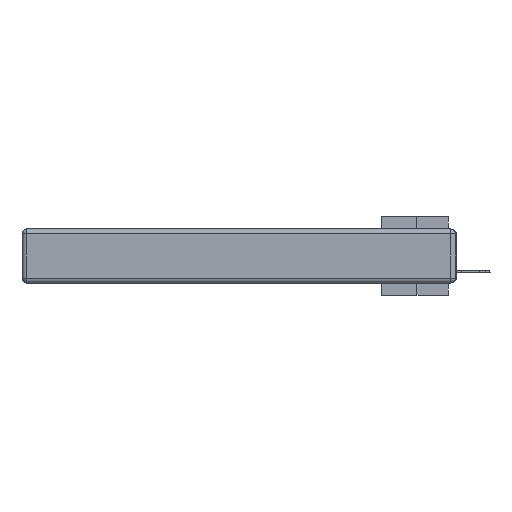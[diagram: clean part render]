
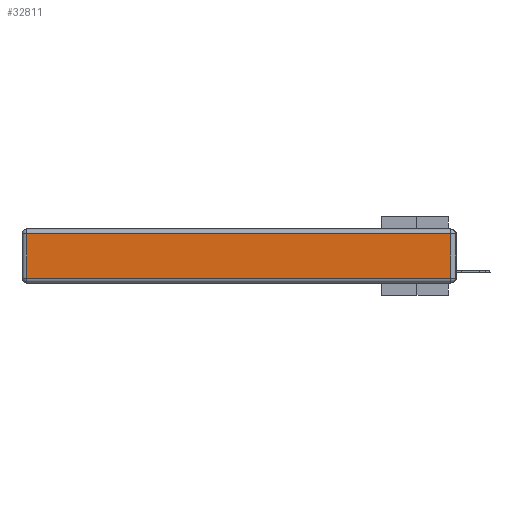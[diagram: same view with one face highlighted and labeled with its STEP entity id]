
A CAD part, left-side view. The second image highlights one B-rep face of the part: STEP entity #32811.
In plain terms, the highlighted planar face has unit normal (-1, 0, 0).
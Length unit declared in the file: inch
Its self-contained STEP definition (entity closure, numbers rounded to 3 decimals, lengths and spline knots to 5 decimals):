
#587 = ORIENTED_EDGE ( 'NONE', *, *, #30968, .T. ) ;
#1299 = EDGE_LOOP ( 'NONE', ( #3835, #18784, #19781, #587 ) ) ;
#2962 = CARTESIAN_POINT ( 'NONE',  ( 0., 0.03, -0.03 ) ) ;
#3835 = ORIENTED_EDGE ( 'NONE', *, *, #29641, .T. ) ;
#3884 = VERTEX_POINT ( 'NONE', #15268 ) ;
#4155 = LINE ( 'NONE', #10941, #34475 ) ;
#4828 = EDGE_CURVE ( 'NONE', #31026, #12802, #4155, .T. ) ;
#4830 = VECTOR ( 'NONE', #8512, 39.37008 ) ;
#5621 = EDGE_CURVE ( 'NONE', #3884, #31026, #7316, .T. ) ;
#7316 = LINE ( 'NONE', #24597, #7793 ) ;
#7793 = VECTOR ( 'NONE', #30874, 39.37008 ) ;
#8512 = DIRECTION ( 'NONE',  ( 0., -1., 0. ) ) ;
#8886 = CARTESIAN_POINT ( 'NONE',  ( 0., 0., -0.313 ) ) ;
#9136 = PLANE ( 'NONE',  #17947 ) ;
#10783 = LINE ( 'NONE', #8886, #4830 ) ;
#10941 = CARTESIAN_POINT ( 'NONE',  ( 0., 2.75, -0.03 ) ) ;
#12802 = VERTEX_POINT ( 'NONE', #35572 ) ;
#13892 = VECTOR ( 'NONE', #23883, 39.37008 ) ;
#13922 = VERTEX_POINT ( 'NONE', #28902 ) ;
#14684 = DIRECTION ( 'NONE',  ( 0., 0., 1. ) ) ;
#15268 = CARTESIAN_POINT ( 'NONE',  ( 0., 0.03, -0.313 ) ) ;
#16967 = DIRECTION ( 'NONE',  ( 0., 1., 0. ) ) ;
#17947 = AXIS2_PLACEMENT_3D ( 'NONE', #32385, #26632, #14684 ) ;
#18784 = ORIENTED_EDGE ( 'NONE', *, *, #5621, .T. ) ;
#19781 = ORIENTED_EDGE ( 'NONE', *, *, #4828, .T. ) ;
#23883 = DIRECTION ( 'NONE',  ( 0., 0., -1. ) ) ;
#24597 = CARTESIAN_POINT ( 'NONE',  ( 0., 0.03, -0.343 ) ) ;
#26632 = DIRECTION ( 'NONE',  ( -1., 0., 0. ) ) ;
#28902 = CARTESIAN_POINT ( 'NONE',  ( 0., 2.72, -0.313 ) ) ;
#29476 = LINE ( 'NONE', #35077, #13892 ) ;
#29641 = EDGE_CURVE ( 'NONE', #13922, #3884, #10783, .T. ) ;
#30874 = DIRECTION ( 'NONE',  ( 0., 0., 1. ) ) ;
#30968 = EDGE_CURVE ( 'NONE', #12802, #13922, #29476, .T. ) ;
#31026 = VERTEX_POINT ( 'NONE', #2962 ) ;
#32385 = CARTESIAN_POINT ( 'NONE',  ( 0., 0., -0.343 ) ) ;
#32811 = ADVANCED_FACE ( 'NONE', ( #35042 ), #9136, .T. ) ;
#34475 = VECTOR ( 'NONE', #16967, 39.37008 ) ;
#35042 = FACE_OUTER_BOUND ( 'NONE', #1299, .T. ) ;
#35077 = CARTESIAN_POINT ( 'NONE',  ( 0., 2.72, -0.343 ) ) ;
#35572 = CARTESIAN_POINT ( 'NONE',  ( 0., 2.72, -0.03 ) ) ;
